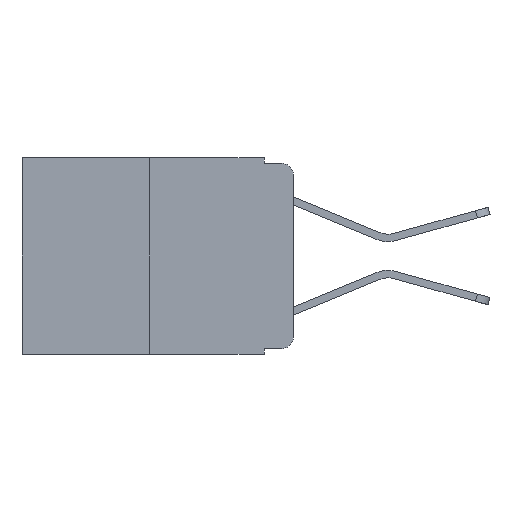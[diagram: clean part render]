
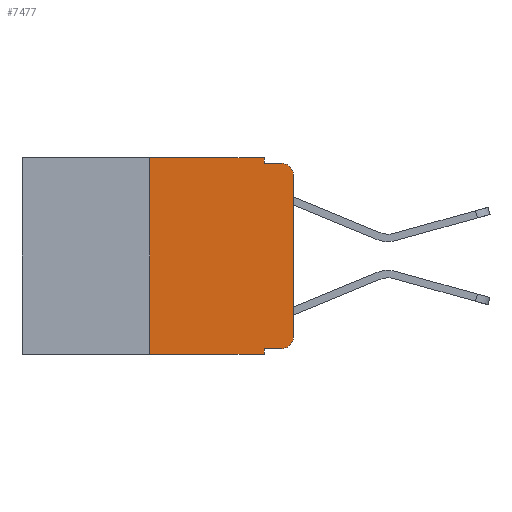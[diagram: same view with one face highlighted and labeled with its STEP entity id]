
A CAD part, left-side view. The second image highlights one B-rep face of the part: STEP entity #7477.
In plain terms, the highlighted planar face has unit normal (-1, 0, 0).
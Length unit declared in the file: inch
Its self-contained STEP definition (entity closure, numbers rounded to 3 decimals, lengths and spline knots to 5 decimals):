
#1 = PLANE ( 'NONE',  #343 ) ;
#99 = VECTOR ( 'NONE', #161, 39.37008 ) ;
#161 = DIRECTION ( 'NONE',  ( 0., 0., 1. ) ) ;
#343 = AXIS2_PLACEMENT_3D ( 'NONE', #3735, #6294, #1032 ) ;
#344 = CARTESIAN_POINT ( 'NONE',  ( 0., 0.051, 0. ) ) ;
#415 = VERTEX_POINT ( 'NONE', #7371 ) ;
#430 = CARTESIAN_POINT ( 'NONE',  ( 0., 0.051, 0. ) ) ;
#908 = DIRECTION ( 'NONE',  ( 0., 0., -1. ) ) ;
#1026 = FACE_OUTER_BOUND ( 'NONE', #6392, .T. ) ;
#1032 = DIRECTION ( 'NONE',  ( 0., 0., -1. ) ) ;
#1262 = DIRECTION ( 'NONE',  ( 0., 0., -1. ) ) ;
#1552 = CARTESIAN_POINT ( 'NONE',  ( 0., 0., -0.03 ) ) ;
#1664 = CARTESIAN_POINT ( 'NONE',  ( 0., 0.25, -0.343 ) ) ;
#1674 = EDGE_CURVE ( 'NONE', #3443, #1961, #3721, .T. ) ;
#1677 = CARTESIAN_POINT ( 'NONE',  ( 0., 0.25, 0. ) ) ;
#1694 = VERTEX_POINT ( 'NONE', #11160 ) ;
#1717 = CARTESIAN_POINT ( 'NONE',  ( 0., 0., 0. ) ) ;
#1817 = VECTOR ( 'NONE', #2609, 39.37008 ) ;
#1961 = VERTEX_POINT ( 'NONE', #5876 ) ;
#2088 = LINE ( 'NONE', #9805, #2374 ) ;
#2122 = LINE ( 'NONE', #8364, #1817 ) ;
#2374 = VECTOR ( 'NONE', #6444, 39.37008 ) ;
#2436 = VERTEX_POINT ( 'NONE', #9748 ) ;
#2453 = ORIENTED_EDGE ( 'NONE', *, *, #4032, .F. ) ;
#2461 = CARTESIAN_POINT ( 'NONE',  ( 0., 0.02, -0.03 ) ) ;
#2609 = DIRECTION ( 'NONE',  ( 0., -1., 0. ) ) ;
#2631 = AXIS2_PLACEMENT_3D ( 'NONE', #2461, #8360, #3344 ) ;
#2826 = CIRCLE ( 'NONE', #3325, 0.02 ) ;
#3008 = EDGE_CURVE ( 'NONE', #2436, #1694, #8907, .T. ) ;
#3264 = VERTEX_POINT ( 'NONE', #1552 ) ;
#3303 = ORIENTED_EDGE ( 'NONE', *, *, #1674, .T. ) ;
#3325 = AXIS2_PLACEMENT_3D ( 'NONE', #5419, #7020, #7010 ) ;
#3344 = DIRECTION ( 'NONE',  ( 0., 0., -1. ) ) ;
#3443 = VERTEX_POINT ( 'NONE', #1664 ) ;
#3542 = DIRECTION ( 'NONE',  ( 0., 0., 1. ) ) ;
#3616 = VERTEX_POINT ( 'NONE', #7165 ) ;
#3721 = LINE ( 'NONE', #4710, #5968 ) ;
#3735 = CARTESIAN_POINT ( 'NONE',  ( 0., 0.473, 0. ) ) ;
#3813 = DIRECTION ( 'NONE',  ( 0., -1., 0. ) ) ;
#4032 = EDGE_CURVE ( 'NONE', #9541, #1961, #10605, .T. ) ;
#4215 = VECTOR ( 'NONE', #1262, 39.37008 ) ;
#4380 = EDGE_CURVE ( 'NONE', #3443, #5057, #7202, .T. ) ;
#4463 = EDGE_CURVE ( 'NONE', #1694, #6995, #2122, .T. ) ;
#4561 = ORIENTED_EDGE ( 'NONE', *, *, #4380, .F. ) ;
#4710 = CARTESIAN_POINT ( 'NONE',  ( 0., 0.473, -0.343 ) ) ;
#5057 = VERTEX_POINT ( 'NONE', #9684 ) ;
#5131 = LINE ( 'NONE', #1717, #7303 ) ;
#5193 = ORIENTED_EDGE ( 'NONE', *, *, #5351, .T. ) ;
#5351 = EDGE_CURVE ( 'NONE', #3616, #415, #2826, .T. ) ;
#5419 = CARTESIAN_POINT ( 'NONE',  ( 0., 0.02, -0.313 ) ) ;
#5732 = ORIENTED_EDGE ( 'NONE', *, *, #10631, .T. ) ;
#5816 = CIRCLE ( 'NONE', #2631, 0.02 ) ;
#5876 = CARTESIAN_POINT ( 'NONE',  ( 0., 0.051, -0.343 ) ) ;
#5968 = VECTOR ( 'NONE', #9770, 39.37008 ) ;
#6294 = DIRECTION ( 'NONE',  ( 1., 0., 0. ) ) ;
#6392 = EDGE_LOOP ( 'NONE', ( #9880, #9926, #9948, #10795, #6823, #4561, #3303, #2453, #5732, #5193 ) ) ;
#6444 = DIRECTION ( 'NONE',  ( 0., -1., 0. ) ) ;
#6478 = CARTESIAN_POINT ( 'NONE',  ( 0., 0.051, -0.333 ) ) ;
#6823 = ORIENTED_EDGE ( 'NONE', *, *, #7622, .F. ) ;
#6995 = VERTEX_POINT ( 'NONE', #8954 ) ;
#7010 = DIRECTION ( 'NONE',  ( 0., 0., -1. ) ) ;
#7020 = DIRECTION ( 'NONE',  ( -1., 0., 0. ) ) ;
#7165 = CARTESIAN_POINT ( 'NONE',  ( 0., 0.02, -0.333 ) ) ;
#7202 = LINE ( 'NONE', #1677, #99 ) ;
#7302 = EDGE_CURVE ( 'NONE', #415, #3264, #5131, .T. ) ;
#7303 = VECTOR ( 'NONE', #3542, 39.37008 ) ;
#7371 = CARTESIAN_POINT ( 'NONE',  ( 0., 0., -0.313 ) ) ;
#7477 = ADVANCED_FACE ( 'NONE', ( #1026 ), #1, .F. ) ;
#7622 = EDGE_CURVE ( 'NONE', #5057, #2436, #2088, .T. ) ;
#8095 = VECTOR ( 'NONE', #908, 39.37008 ) ;
#8360 = DIRECTION ( 'NONE',  ( -1., 0., 0. ) ) ;
#8364 = CARTESIAN_POINT ( 'NONE',  ( 0., 0.051, -0.01 ) ) ;
#8380 = LINE ( 'NONE', #9659, #10629 ) ;
#8907 = LINE ( 'NONE', #344, #4215 ) ;
#8954 = CARTESIAN_POINT ( 'NONE',  ( 0., 0.02, -0.01 ) ) ;
#9541 = VERTEX_POINT ( 'NONE', #6478 ) ;
#9659 = CARTESIAN_POINT ( 'NONE',  ( 0., 0.051, -0.333 ) ) ;
#9684 = CARTESIAN_POINT ( 'NONE',  ( 0., 0.25, 0. ) ) ;
#9748 = CARTESIAN_POINT ( 'NONE',  ( 0., 0.051, 0. ) ) ;
#9770 = DIRECTION ( 'NONE',  ( 0., -1., 0. ) ) ;
#9805 = CARTESIAN_POINT ( 'NONE',  ( 0., 0.473, 0. ) ) ;
#9880 = ORIENTED_EDGE ( 'NONE', *, *, #7302, .T. ) ;
#9926 = ORIENTED_EDGE ( 'NONE', *, *, #10930, .T. ) ;
#9948 = ORIENTED_EDGE ( 'NONE', *, *, #4463, .F. ) ;
#10605 = LINE ( 'NONE', #430, #8095 ) ;
#10629 = VECTOR ( 'NONE', #3813, 39.37008 ) ;
#10631 = EDGE_CURVE ( 'NONE', #9541, #3616, #8380, .T. ) ;
#10795 = ORIENTED_EDGE ( 'NONE', *, *, #3008, .F. ) ;
#10930 = EDGE_CURVE ( 'NONE', #3264, #6995, #5816, .T. ) ;
#11160 = CARTESIAN_POINT ( 'NONE',  ( 0., 0.051, -0.01 ) ) ;
